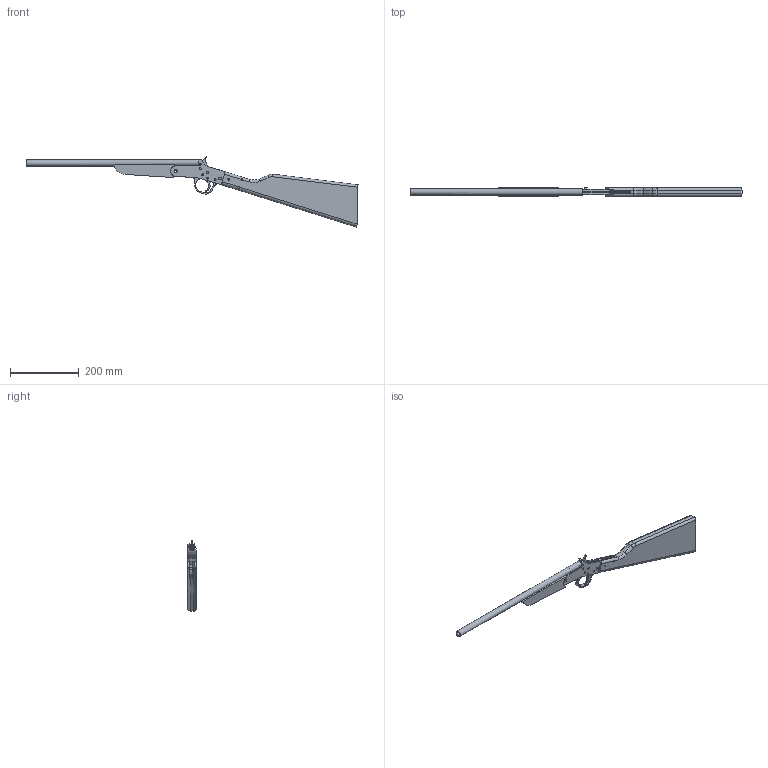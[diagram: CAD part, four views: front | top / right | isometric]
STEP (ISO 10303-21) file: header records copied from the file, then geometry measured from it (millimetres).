
FILE_DESCRIPTION(/* description */ ('STEP AP214'),/* implementation_level */ '2;1');
FILE_NAME(/* name */ '2-home made 410.step',/* time_stamp */ '2024-01-14T22:06:41+05:00',/* author */ ('ASDAFF'),/* organization */ (' '),/* preprocessor_version */ 'ST-DEVELOPER v18.1',/* originating_system */ 'Autodesk Inventor 2022',/* authorisation */ ' ');
FILE_SCHEMA (('AUTOMOTIVE_DESIGN { 1 0 10303 214 3 1 1 }'));
Length unit declared in the file: millimetre
Products named in the file (37): 2-home made 410; Рамка; Body; StockHolder; Body Geometry; springs; Pin; DownFill; Stock; Stock Geometry; Pin2; Trig_support; Point2B; Mover; Mover Geometry; Ствол; Outer; Outer Geometry; Wood; Bolet; Bolet Geometry; body2; G; Opener; Opener Geometry; pin3; Opener_Trig; Mount; 1; Spring_Dazy_norm2; Spring_Dazy_norm2 Geometry; Pins; Pins Geometry; Vasher; Fireed; Спусковой крючок; Hammer
Assembly tree (36 placements, depth 5):
  2-home made 410
    Рамка
      Body
        StockHolder
        Body Geometry
        springs
      Pin
      DownFill
      Stock
        Stock Geometry
        Pin2
      Trig_support
      Point2B
    Mover
      Mover Geometry
      Ствол
      Outer
        Outer Geometry
      Wood
      Bolet
        Bolet Geometry
        body2
        G
    Opener
      Opener Geometry
      pin3
      Opener_Trig
    Mount
    1
      Spring_Dazy_norm2
        Spring_Dazy_norm2 Geometry
        Pins
          Pins Geometry
          Vasher
        Fireed
      Спусковой крючок
      Hammer
Bounding box: 964.54 x 25 x 204.48 mm (x, y, z)
Volume: 1045713 mm3; surface area: 216068.6 mm2
Topology: 38 solids, 38 shells, 320 faces, 732 edges, 490 vertices
Faces by surface type: plane 168, cylinder 118, bspline 26, torus 8
Full cylindrical faces by diameter (mm): 0.7 x2, 1 x2, 2.3 x1, 2.5 x3, 2.76 x1, 2.8 x1, 2.96 x2, 3 x1, 3.8 x1, 3.994 x1, 4 x3, 4.058 x4, 4.5 x1, 5 x18, 5.073 x4, 5.36 x1, 8 x2, 8.026 x2, 8.116 x2, 9 x2, 11 x2, 12 x3, 13.6 x1, 18 x1
Entity records: 26329 total; most frequent: CARTESIAN_POINT 17314, DIRECTION 1711, ORIENTED_EDGE 1464, EDGE_CURVE 732, AXIS2_PLACEMENT_3D 662, VERTEX_POINT 490, EDGE_LOOP 388, LINE 387
